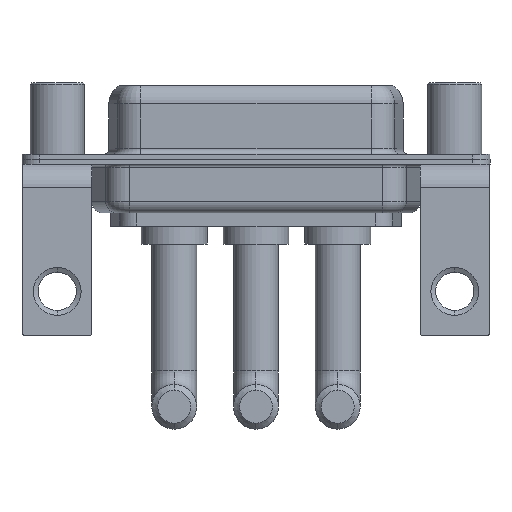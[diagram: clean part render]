
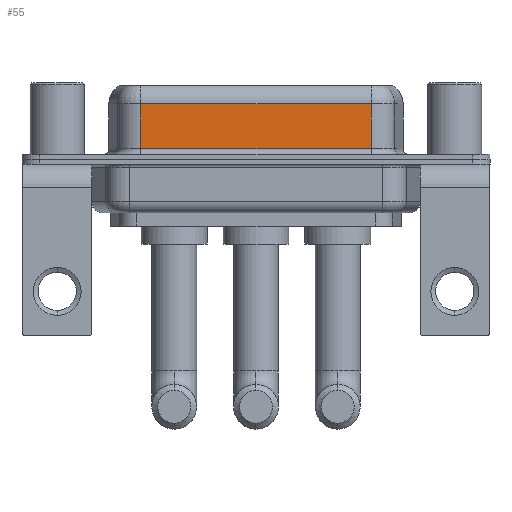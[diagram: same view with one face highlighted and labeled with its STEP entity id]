
A CAD part, front view. The second image highlights one B-rep face of the part: STEP entity #55.
In plain terms, the highlighted planar face has unit normal (0, -1, 0).
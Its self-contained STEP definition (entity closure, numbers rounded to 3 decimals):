
#55 = ADVANCED_FACE ( 'NONE', ( #6403 ), #7450, .F. ) ;
#67 = LINE ( 'NONE', #1109, #4046 ) ;
#155 = CARTESIAN_POINT ( 'NONE',  ( 7.013, -3.95, 4.65 ) ) ;
#368 = VERTEX_POINT ( 'NONE', #155 ) ;
#417 = EDGE_CURVE ( 'NONE', #7625, #3933, #7227, .T. ) ;
#434 = DIRECTION ( 'NONE',  ( 0., 0., -1. ) ) ;
#1039 = DIRECTION ( 'NONE',  ( -1., 0., 0. ) ) ;
#1109 = CARTESIAN_POINT ( 'NONE',  ( 7.013, -3.95, 6.4 ) ) ;
#1135 = DIRECTION ( 'NONE',  ( 1., 0., 0. ) ) ;
#2312 = ORIENTED_EDGE ( 'NONE', *, *, #417, .F. ) ;
#2589 = EDGE_CURVE ( 'NONE', #7625, #368, #5653, .T. ) ;
#2627 = ORIENTED_EDGE ( 'NONE', *, *, #2589, .T. ) ;
#2667 = ORIENTED_EDGE ( 'NONE', *, *, #13244, .T. ) ;
#3933 = VERTEX_POINT ( 'NONE', #6373 ) ;
#4046 = VECTOR ( 'NONE', #13676, 1000. ) ;
#5653 = LINE ( 'NONE', #11507, #13867 ) ;
#6142 = VECTOR ( 'NONE', #434, 1000. ) ;
#6373 = CARTESIAN_POINT ( 'NONE',  ( 26.287, -3.95, 0.9 ) ) ;
#6403 = FACE_OUTER_BOUND ( 'NONE', #9065, .T. ) ;
#6932 = LINE ( 'NONE', #10247, #7636 ) ;
#7227 = LINE ( 'NONE', #11816, #6142 ) ;
#7450 = PLANE ( 'NONE',  #14279 ) ;
#7625 = VERTEX_POINT ( 'NONE', #9257 ) ;
#7636 = VECTOR ( 'NONE', #1135, 1000. ) ;
#8718 = DIRECTION ( 'NONE',  ( 0., 0., 1. ) ) ;
#9065 = EDGE_LOOP ( 'NONE', ( #2312, #2627, #10863, #2667 ) ) ;
#9257 = CARTESIAN_POINT ( 'NONE',  ( 26.287, -3.95, 4.65 ) ) ;
#10108 = EDGE_CURVE ( 'NONE', #368, #14301, #67, .T. ) ;
#10247 = CARTESIAN_POINT ( 'NONE',  ( 26.287, -3.95, 0.9 ) ) ;
#10863 = ORIENTED_EDGE ( 'NONE', *, *, #10108, .T. ) ;
#11073 = DIRECTION ( 'NONE',  ( 0., 1., 0. ) ) ;
#11507 = CARTESIAN_POINT ( 'NONE',  ( 26.287, -3.95, 4.65 ) ) ;
#11816 = CARTESIAN_POINT ( 'NONE',  ( 26.287, -3.95, 6.4 ) ) ;
#13244 = EDGE_CURVE ( 'NONE', #14301, #3933, #6932, .T. ) ;
#13676 = DIRECTION ( 'NONE',  ( 0., 0., -1. ) ) ;
#13741 = CARTESIAN_POINT ( 'NONE',  ( 7.013, -3.95, 0.9 ) ) ;
#13867 = VECTOR ( 'NONE', #1039, 1000. ) ;
#14279 = AXIS2_PLACEMENT_3D ( 'NONE', #14451, #11073, #8718 ) ;
#14301 = VERTEX_POINT ( 'NONE', #13741 ) ;
#14451 = CARTESIAN_POINT ( 'NONE',  ( 26.287, -3.95, 6.4 ) ) ;
